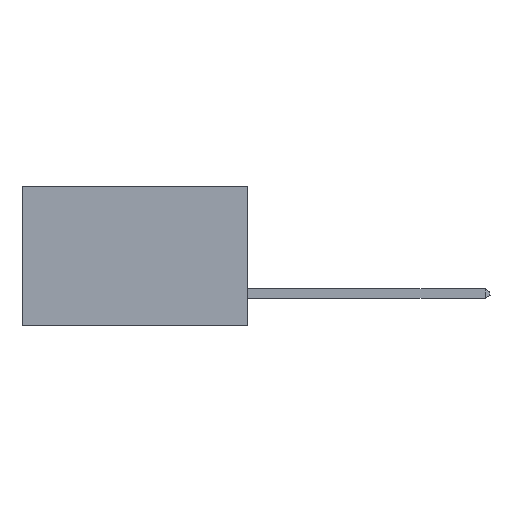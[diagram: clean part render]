
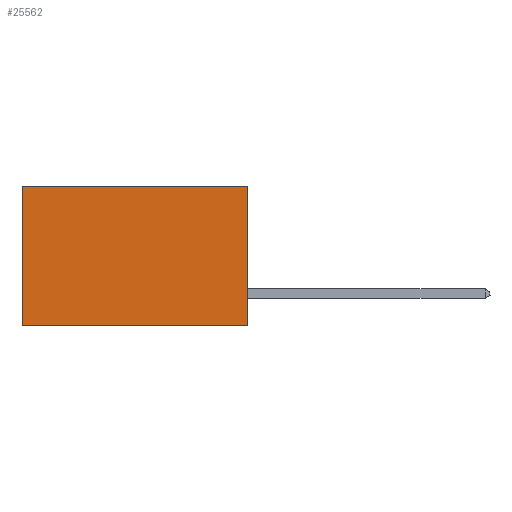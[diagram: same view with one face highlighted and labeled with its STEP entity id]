
A CAD part, left-side view. The second image highlights one B-rep face of the part: STEP entity #25562.
In plain terms, the highlighted planar face has unit normal (-1, 0, 0).
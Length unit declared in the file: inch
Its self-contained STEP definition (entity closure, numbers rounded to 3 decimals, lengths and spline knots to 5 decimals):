
#1535 = VERTEX_POINT ( 'NONE', #16792 ) ;
#1559 = CARTESIAN_POINT ( 'NONE',  ( 0.298, 0.6, -0.37 ) ) ;
#2202 = CARTESIAN_POINT ( 'NONE',  ( 0.298, 0.6, 0. ) ) ;
#2529 = PLANE ( 'NONE',  #20931 ) ;
#6471 = CARTESIAN_POINT ( 'NONE',  ( 0.298, 0., 0. ) ) ;
#8006 = EDGE_CURVE ( 'NONE', #13001, #10614, #20050, .T. ) ;
#8331 = CARTESIAN_POINT ( 'NONE',  ( 0.298, 0., -0.37 ) ) ;
#8803 = CARTESIAN_POINT ( 'NONE',  ( 0.298, 0.6, 0. ) ) ;
#10614 = VERTEX_POINT ( 'NONE', #1559 ) ;
#10812 = DIRECTION ( 'NONE',  ( 0., 1., 0. ) ) ;
#10878 = LINE ( 'NONE', #22855, #13706 ) ;
#11860 = VECTOR ( 'NONE', #19123, 39.37008 ) ;
#11944 = ORIENTED_EDGE ( 'NONE', *, *, #8006, .T. ) ;
#12432 = DIRECTION ( 'NONE',  ( 1., 0., 0. ) ) ;
#13001 = VERTEX_POINT ( 'NONE', #8803 ) ;
#13706 = VECTOR ( 'NONE', #10812, 39.37008 ) ;
#14317 = DIRECTION ( 'NONE',  ( 0., 0., -1. ) ) ;
#14558 = LINE ( 'NONE', #18144, #25510 ) ;
#16127 = DIRECTION ( 'NONE',  ( 0., 0., -1. ) ) ;
#16212 = EDGE_CURVE ( 'NONE', #22603, #10614, #17847, .T. ) ;
#16275 = ORIENTED_EDGE ( 'NONE', *, *, #19304, .F. ) ;
#16792 = CARTESIAN_POINT ( 'NONE',  ( 0.298, 0., 0. ) ) ;
#17847 = LINE ( 'NONE', #8331, #11860 ) ;
#18144 = CARTESIAN_POINT ( 'NONE',  ( 0.298, 0., 0. ) ) ;
#19123 = DIRECTION ( 'NONE',  ( 0., 1., 0. ) ) ;
#19304 = EDGE_CURVE ( 'NONE', #1535, #22603, #14558, .T. ) ;
#19401 = VECTOR ( 'NONE', #25921, 39.37008 ) ;
#20050 = LINE ( 'NONE', #2202, #19401 ) ;
#20931 = AXIS2_PLACEMENT_3D ( 'NONE', #6471, #12432, #14317 ) ;
#22603 = VERTEX_POINT ( 'NONE', #25973 ) ;
#22855 = CARTESIAN_POINT ( 'NONE',  ( 0.298, 0., 0. ) ) ;
#22880 = EDGE_LOOP ( 'NONE', ( #11944, #22901, #16275, #23990 ) ) ;
#22901 = ORIENTED_EDGE ( 'NONE', *, *, #16212, .F. ) ;
#23990 = ORIENTED_EDGE ( 'NONE', *, *, #25029, .T. ) ;
#25029 = EDGE_CURVE ( 'NONE', #1535, #13001, #10878, .T. ) ;
#25510 = VECTOR ( 'NONE', #16127, 39.37008 ) ;
#25562 = ADVANCED_FACE ( 'NONE', ( #25932 ), #2529, .F. ) ;
#25921 = DIRECTION ( 'NONE',  ( 0., 0., -1. ) ) ;
#25932 = FACE_OUTER_BOUND ( 'NONE', #22880, .T. ) ;
#25973 = CARTESIAN_POINT ( 'NONE',  ( 0.298, 0., -0.37 ) ) ;
